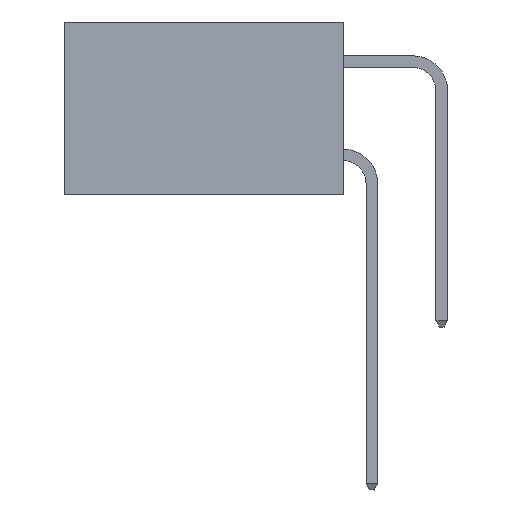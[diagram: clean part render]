
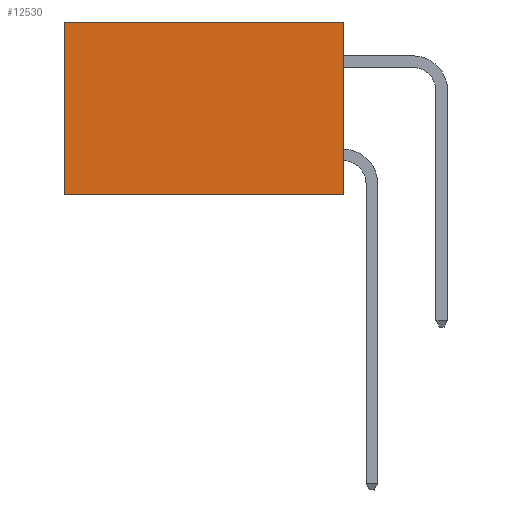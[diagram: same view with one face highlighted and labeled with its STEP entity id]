
A CAD part, left-side view. The second image highlights one B-rep face of the part: STEP entity #12530.
In plain terms, the highlighted planar face has unit normal (-1, 0, 0).
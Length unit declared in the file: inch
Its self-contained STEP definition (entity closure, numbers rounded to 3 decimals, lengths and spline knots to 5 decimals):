
#217 = CARTESIAN_POINT ( 'NONE',  ( 0.298, 0., 0. ) ) ;
#1117 = AXIS2_PLACEMENT_3D ( 'NONE', #12548, #6344, #13576 ) ;
#1274 = VERTEX_POINT ( 'NONE', #8067 ) ;
#1400 = DIRECTION ( 'NONE',  ( 0., 1., 0. ) ) ;
#1508 = ORIENTED_EDGE ( 'NONE', *, *, #9926, .F. ) ;
#1569 = ORIENTED_EDGE ( 'NONE', *, *, #7754, .T. ) ;
#2087 = VECTOR ( 'NONE', #3071, 39.37008 ) ;
#2089 = ORIENTED_EDGE ( 'NONE', *, *, #2947, .F. ) ;
#2802 = VECTOR ( 'NONE', #12191, 39.37008 ) ;
#2947 = EDGE_CURVE ( 'NONE', #5765, #8202, #5831, .T. ) ;
#3071 = DIRECTION ( 'NONE',  ( 0., 0., -1. ) ) ;
#3834 = CARTESIAN_POINT ( 'NONE',  ( 0.298, 0., 0. ) ) ;
#5765 = VERTEX_POINT ( 'NONE', #11766 ) ;
#5831 = LINE ( 'NONE', #3834, #2802 ) ;
#6119 = CARTESIAN_POINT ( 'NONE',  ( 0.298, 0.6, 0. ) ) ;
#6344 = DIRECTION ( 'NONE',  ( 1., 0., 0. ) ) ;
#7754 = EDGE_CURVE ( 'NONE', #1274, #9103, #8028, .T. ) ;
#7815 = VECTOR ( 'NONE', #8534, 39.37008 ) ;
#8028 = LINE ( 'NONE', #6119, #2087 ) ;
#8067 = CARTESIAN_POINT ( 'NONE',  ( 0.298, 0.6, 0. ) ) ;
#8148 = LINE ( 'NONE', #10616, #7815 ) ;
#8202 = VERTEX_POINT ( 'NONE', #10746 ) ;
#8249 = LINE ( 'NONE', #217, #13589 ) ;
#8534 = DIRECTION ( 'NONE',  ( 0., 1., 0. ) ) ;
#9103 = VERTEX_POINT ( 'NONE', #11145 ) ;
#9926 = EDGE_CURVE ( 'NONE', #8202, #9103, #8148, .T. ) ;
#10487 = PLANE ( 'NONE',  #1117 ) ;
#10616 = CARTESIAN_POINT ( 'NONE',  ( 0.298, 0., -0.37 ) ) ;
#10705 = EDGE_LOOP ( 'NONE', ( #1569, #1508, #2089, #11967 ) ) ;
#10746 = CARTESIAN_POINT ( 'NONE',  ( 0.298, 0., -0.37 ) ) ;
#11145 = CARTESIAN_POINT ( 'NONE',  ( 0.298, 0.6, -0.37 ) ) ;
#11766 = CARTESIAN_POINT ( 'NONE',  ( 0.298, 0., 0. ) ) ;
#11967 = ORIENTED_EDGE ( 'NONE', *, *, #12367, .T. ) ;
#12191 = DIRECTION ( 'NONE',  ( 0., 0., -1. ) ) ;
#12367 = EDGE_CURVE ( 'NONE', #5765, #1274, #8249, .T. ) ;
#12530 = ADVANCED_FACE ( 'NONE', ( #12672 ), #10487, .F. ) ;
#12548 = CARTESIAN_POINT ( 'NONE',  ( 0.298, 0., 0. ) ) ;
#12672 = FACE_OUTER_BOUND ( 'NONE', #10705, .T. ) ;
#13576 = DIRECTION ( 'NONE',  ( 0., 0., -1. ) ) ;
#13589 = VECTOR ( 'NONE', #1400, 39.37008 ) ;
